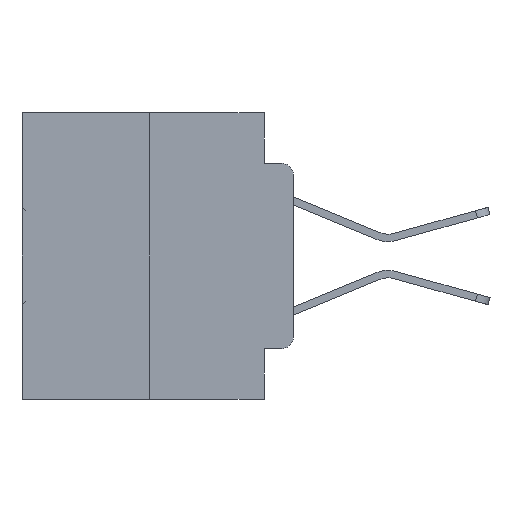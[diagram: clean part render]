
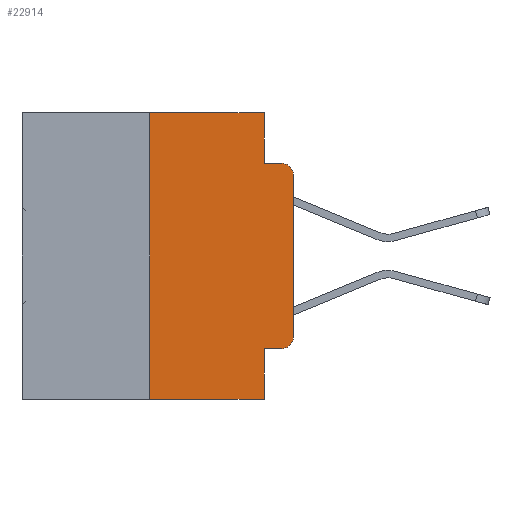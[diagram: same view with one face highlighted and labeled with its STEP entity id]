
A CAD part, left-side view. The second image highlights one B-rep face of the part: STEP entity #22914.
In plain terms, the highlighted planar face has unit normal (-1, 0, 0).
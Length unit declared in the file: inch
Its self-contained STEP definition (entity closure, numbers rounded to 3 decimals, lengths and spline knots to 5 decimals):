
#861 = EDGE_CURVE ( 'NONE', #23212, #28183, #24165, .T. ) ;
#989 = LINE ( 'NONE', #18503, #14908 ) ;
#1146 = CARTESIAN_POINT ( 'NONE',  ( 0., 0.051, 0. ) ) ;
#2058 = CARTESIAN_POINT ( 'NONE',  ( 0., 0., -0.1085 ) ) ;
#2186 = ORIENTED_EDGE ( 'NONE', *, *, #20119, .F. ) ;
#2604 = ORIENTED_EDGE ( 'NONE', *, *, #23903, .T. ) ;
#2806 = FACE_OUTER_BOUND ( 'NONE', #30780, .T. ) ;
#3126 = EDGE_CURVE ( 'NONE', #31261, #30289, #24036, .T. ) ;
#3477 = CARTESIAN_POINT ( 'NONE',  ( 0., 0.051, -0.0885 ) ) ;
#3738 = DIRECTION ( 'NONE',  ( 0., 0., -1. ) ) ;
#4016 = DIRECTION ( 'NONE',  ( 0., -1., 0. ) ) ;
#4538 = CIRCLE ( 'NONE', #29408, 0.02 ) ;
#4636 = EDGE_CURVE ( 'NONE', #10281, #23212, #19840, .T. ) ;
#4907 = VERTEX_POINT ( 'NONE', #7460 ) ;
#5007 = LINE ( 'NONE', #31811, #9285 ) ;
#5104 = DIRECTION ( 'NONE',  ( 0., -1., 0. ) ) ;
#5997 = VERTEX_POINT ( 'NONE', #18245 ) ;
#6390 = VECTOR ( 'NONE', #3738, 39.37008 ) ;
#6584 = CARTESIAN_POINT ( 'NONE',  ( 0., 0.25, 0. ) ) ;
#6675 = VERTEX_POINT ( 'NONE', #11798 ) ;
#7460 = CARTESIAN_POINT ( 'NONE',  ( 0., 0.02, -0.4115 ) ) ;
#7791 = ORIENTED_EDGE ( 'NONE', *, *, #10322, .F. ) ;
#8543 = VECTOR ( 'NONE', #27728, 39.37008 ) ;
#8802 = CARTESIAN_POINT ( 'NONE',  ( 0., 0.051, -0.5 ) ) ;
#9285 = VECTOR ( 'NONE', #4016, 39.37008 ) ;
#9340 = EDGE_CURVE ( 'NONE', #4907, #10281, #4538, .T. ) ;
#9954 = EDGE_CURVE ( 'NONE', #6675, #5997, #27090, .T. ) ;
#10281 = VERTEX_POINT ( 'NONE', #19245 ) ;
#10322 = EDGE_CURVE ( 'NONE', #17659, #32542, #22291, .T. ) ;
#10349 = CARTESIAN_POINT ( 'NONE',  ( 0., 0.02, -0.0885 ) ) ;
#11091 = EDGE_CURVE ( 'NONE', #5997, #31261, #31803, .T. ) ;
#11151 = VECTOR ( 'NONE', #21758, 39.37008 ) ;
#11419 = DIRECTION ( 'NONE',  ( 0., 0., 1. ) ) ;
#11798 = CARTESIAN_POINT ( 'NONE',  ( 0., 0.25, -0.5 ) ) ;
#12390 = CARTESIAN_POINT ( 'NONE',  ( 0., 0.051, 0. ) ) ;
#12470 = DIRECTION ( 'NONE',  ( -1., 0., 0. ) ) ;
#12508 = DIRECTION ( 'NONE',  ( 0., -1., 0. ) ) ;
#13126 = ORIENTED_EDGE ( 'NONE', *, *, #19284, .T. ) ;
#13663 = CARTESIAN_POINT ( 'NONE',  ( 0., 0.02, -0.3915 ) ) ;
#14040 = AXIS2_PLACEMENT_3D ( 'NONE', #21195, #26227, #31759 ) ;
#14662 = VECTOR ( 'NONE', #11419, 39.37008 ) ;
#14908 = VECTOR ( 'NONE', #17943, 39.37008 ) ;
#14993 = DIRECTION ( 'NONE',  ( 0., 0., -1. ) ) ;
#15460 = ORIENTED_EDGE ( 'NONE', *, *, #4636, .T. ) ;
#15998 = DIRECTION ( 'NONE',  ( -1., 0., 0. ) ) ;
#16667 = CARTESIAN_POINT ( 'NONE',  ( 0., 0.051, -0.4115 ) ) ;
#17659 = VERTEX_POINT ( 'NONE', #16667 ) ;
#17739 = ORIENTED_EDGE ( 'NONE', *, *, #861, .T. ) ;
#17943 = DIRECTION ( 'NONE',  ( 0., -1., 0. ) ) ;
#18245 = CARTESIAN_POINT ( 'NONE',  ( 0., 0.25, 0. ) ) ;
#18503 = CARTESIAN_POINT ( 'NONE',  ( 0., 0.473, -0.5 ) ) ;
#18867 = PLANE ( 'NONE',  #14040 ) ;
#19245 = CARTESIAN_POINT ( 'NONE',  ( 0., 0., -0.3915 ) ) ;
#19284 = EDGE_CURVE ( 'NONE', #6675, #32542, #989, .T. ) ;
#19840 = LINE ( 'NONE', #30958, #14662 ) ;
#20119 = EDGE_CURVE ( 'NONE', #30289, #28183, #5007, .T. ) ;
#20494 = ORIENTED_EDGE ( 'NONE', *, *, #3126, .F. ) ;
#21042 = VECTOR ( 'NONE', #5104, 39.37008 ) ;
#21195 = CARTESIAN_POINT ( 'NONE',  ( 0., 0.473, 0. ) ) ;
#21218 = DIRECTION ( 'NONE',  ( 0., 0., -1. ) ) ;
#21758 = DIRECTION ( 'NONE',  ( 0., 0., 1. ) ) ;
#22291 = LINE ( 'NONE', #1146, #6390 ) ;
#22373 = CARTESIAN_POINT ( 'NONE',  ( 0., 0.473, 0. ) ) ;
#22615 = CARTESIAN_POINT ( 'NONE',  ( 0., 0.051, 0. ) ) ;
#22647 = CARTESIAN_POINT ( 'NONE',  ( 0., 0.051, -0.4115 ) ) ;
#22914 = ADVANCED_FACE ( 'NONE', ( #2806 ), #18867, .F. ) ;
#23212 = VERTEX_POINT ( 'NONE', #2058 ) ;
#23737 = VECTOR ( 'NONE', #12508, 39.37008 ) ;
#23903 = EDGE_CURVE ( 'NONE', #17659, #4907, #26944, .T. ) ;
#23916 = AXIS2_PLACEMENT_3D ( 'NONE', #25142, #12470, #14993 ) ;
#24036 = LINE ( 'NONE', #12390, #8543 ) ;
#24165 = CIRCLE ( 'NONE', #23916, 0.02 ) ;
#25142 = CARTESIAN_POINT ( 'NONE',  ( 0., 0.02, -0.1085 ) ) ;
#25622 = ORIENTED_EDGE ( 'NONE', *, *, #11091, .F. ) ;
#26227 = DIRECTION ( 'NONE',  ( 1., 0., 0. ) ) ;
#26944 = LINE ( 'NONE', #22647, #23737 ) ;
#27090 = LINE ( 'NONE', #6584, #11151 ) ;
#27728 = DIRECTION ( 'NONE',  ( 0., 0., -1. ) ) ;
#27774 = ORIENTED_EDGE ( 'NONE', *, *, #9340, .T. ) ;
#28183 = VERTEX_POINT ( 'NONE', #10349 ) ;
#28845 = ORIENTED_EDGE ( 'NONE', *, *, #9954, .F. ) ;
#29408 = AXIS2_PLACEMENT_3D ( 'NONE', #13663, #15998, #21218 ) ;
#30289 = VERTEX_POINT ( 'NONE', #3477 ) ;
#30780 = EDGE_LOOP ( 'NONE', ( #15460, #17739, #2186, #20494, #25622, #28845, #13126, #7791, #2604, #27774 ) ) ;
#30958 = CARTESIAN_POINT ( 'NONE',  ( 0., 0., 0. ) ) ;
#31261 = VERTEX_POINT ( 'NONE', #22615 ) ;
#31759 = DIRECTION ( 'NONE',  ( 0., 0., -1. ) ) ;
#31803 = LINE ( 'NONE', #22373, #21042 ) ;
#31811 = CARTESIAN_POINT ( 'NONE',  ( 0., 0.051, -0.0885 ) ) ;
#32542 = VERTEX_POINT ( 'NONE', #8802 ) ;
